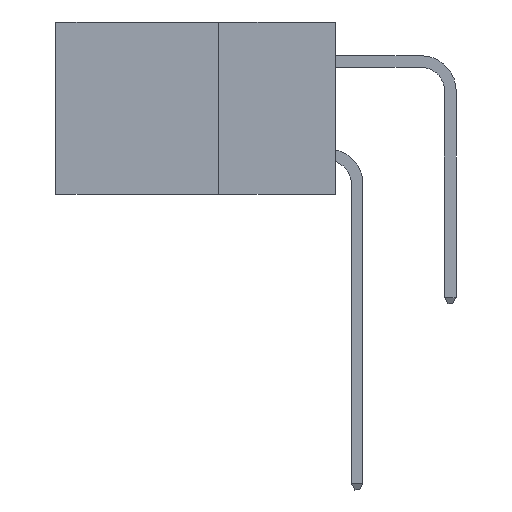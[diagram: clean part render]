
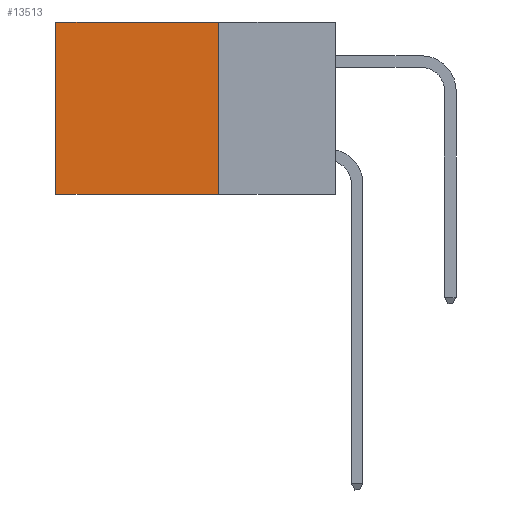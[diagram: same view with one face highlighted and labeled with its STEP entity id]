
A CAD part, left-side view. The second image highlights one B-rep face of the part: STEP entity #13513.
In plain terms, the highlighted planar face has unit normal (-1, 0, 0).
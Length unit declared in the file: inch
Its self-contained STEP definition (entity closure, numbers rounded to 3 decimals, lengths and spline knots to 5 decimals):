
#793 = CARTESIAN_POINT ( 'NONE',  ( 0.2875, 0.6, 0. ) ) ;
#940 = VERTEX_POINT ( 'NONE', #18744 ) ;
#2452 = VERTEX_POINT ( 'NONE', #793 ) ;
#2602 = AXIS2_PLACEMENT_3D ( 'NONE', #19472, #18985, #14059 ) ;
#3509 = ORIENTED_EDGE ( 'NONE', *, *, #18427, .F. ) ;
#4595 = DIRECTION ( 'NONE',  ( 0., 0., -1. ) ) ;
#5443 = VECTOR ( 'NONE', #26780, 39.37008 ) ;
#7017 = CARTESIAN_POINT ( 'NONE',  ( 0.2875, 0.25, -0.37 ) ) ;
#7259 = VECTOR ( 'NONE', #4595, 39.37008 ) ;
#8702 = ORIENTED_EDGE ( 'NONE', *, *, #27509, .F. ) ;
#9623 = CARTESIAN_POINT ( 'NONE',  ( 0.2875, 0.25, 0. ) ) ;
#11217 = EDGE_LOOP ( 'NONE', ( #28041, #3509, #8702, #22431 ) ) ;
#11418 = FACE_OUTER_BOUND ( 'NONE', #11217, .T. ) ;
#11736 = PLANE ( 'NONE',  #2602 ) ;
#11788 = LINE ( 'NONE', #9623, #5443 ) ;
#12017 = LINE ( 'NONE', #29620, #7259 ) ;
#12243 = EDGE_CURVE ( 'NONE', #2452, #940, #12017, .T. ) ;
#13513 = ADVANCED_FACE ( 'NONE', ( #11418 ), #11736, .F. ) ;
#14059 = DIRECTION ( 'NONE',  ( 0., 0., -1. ) ) ;
#14130 = CARTESIAN_POINT ( 'NONE',  ( 0.2875, 0.25, -0.37 ) ) ;
#14499 = VECTOR ( 'NONE', #18669, 39.37008 ) ;
#15877 = LINE ( 'NONE', #28532, #14499 ) ;
#18427 = EDGE_CURVE ( 'NONE', #29782, #940, #27108, .T. ) ;
#18489 = EDGE_CURVE ( 'NONE', #20367, #2452, #11788, .T. ) ;
#18669 = DIRECTION ( 'NONE',  ( 0., 0., -1. ) ) ;
#18744 = CARTESIAN_POINT ( 'NONE',  ( 0.2875, 0.6, -0.37 ) ) ;
#18985 = DIRECTION ( 'NONE',  ( 1., 0., 0. ) ) ;
#19434 = CARTESIAN_POINT ( 'NONE',  ( 0.2875, 0.25, 0. ) ) ;
#19472 = CARTESIAN_POINT ( 'NONE',  ( 0.2875, 0.25, 0. ) ) ;
#20367 = VERTEX_POINT ( 'NONE', #19434 ) ;
#22268 = VECTOR ( 'NONE', #29391, 39.37008 ) ;
#22431 = ORIENTED_EDGE ( 'NONE', *, *, #18489, .T. ) ;
#26780 = DIRECTION ( 'NONE',  ( 0., 1., 0. ) ) ;
#27108 = LINE ( 'NONE', #7017, #22268 ) ;
#27509 = EDGE_CURVE ( 'NONE', #20367, #29782, #15877, .T. ) ;
#28041 = ORIENTED_EDGE ( 'NONE', *, *, #12243, .T. ) ;
#28532 = CARTESIAN_POINT ( 'NONE',  ( 0.2875, 0.25, 0. ) ) ;
#29391 = DIRECTION ( 'NONE',  ( 0., 1., 0. ) ) ;
#29620 = CARTESIAN_POINT ( 'NONE',  ( 0.2875, 0.6, 0. ) ) ;
#29782 = VERTEX_POINT ( 'NONE', #14130 ) ;
